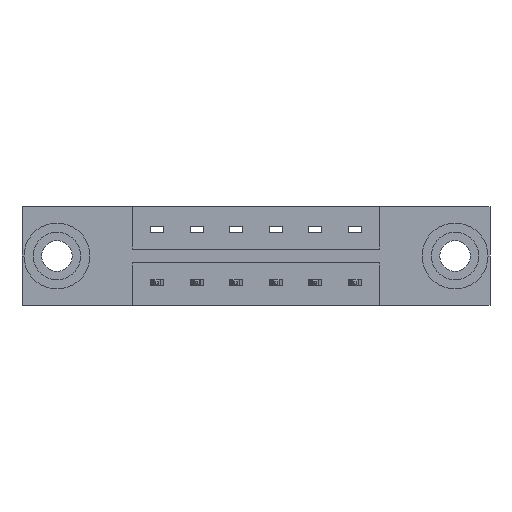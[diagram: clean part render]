
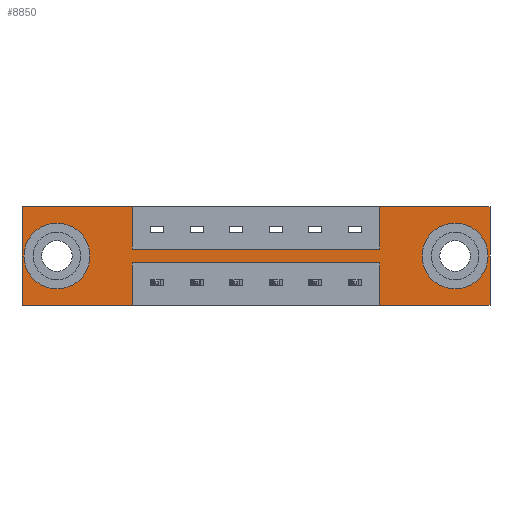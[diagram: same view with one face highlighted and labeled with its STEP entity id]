
A CAD part, front view. The second image highlights one B-rep face of the part: STEP entity #8850.
In plain terms, the highlighted planar face has unit normal (0, -1, 0).
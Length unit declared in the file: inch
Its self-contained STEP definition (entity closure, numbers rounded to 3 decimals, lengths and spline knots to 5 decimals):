
#190 = CARTESIAN_POINT ( 'NONE',  ( 0., 0., -0.375 ) ) ;
#404 = VECTOR ( 'NONE', #4801, 39.37008 ) ;
#410 = CARTESIAN_POINT ( 'NONE',  ( 1.3575, 0., -0.375 ) ) ;
#414 = CARTESIAN_POINT ( 'NONE',  ( 0.1325, 0., -0.2655 ) ) ;
#496 = EDGE_CURVE ( 'NONE', #5405, #872, #3525, .T. ) ;
#663 = CARTESIAN_POINT ( 'NONE',  ( 1.3575, 0., -0.214 ) ) ;
#673 = CIRCLE ( 'NONE', #7568, 0.078 ) ;
#729 = VERTEX_POINT ( 'NONE', #8102 ) ;
#759 = VERTEX_POINT ( 'NONE', #3220 ) ;
#762 = CARTESIAN_POINT ( 'NONE',  ( 1.3575, 0., 0. ) ) ;
#791 = LINE ( 'NONE', #9016, #7398 ) ;
#846 = DIRECTION ( 'NONE',  ( 1., 0., 0. ) ) ;
#872 = VERTEX_POINT ( 'NONE', #1295 ) ;
#899 = CARTESIAN_POINT ( 'NONE',  ( 0.4175, 0., -0.161 ) ) ;
#926 = EDGE_CURVE ( 'NONE', #759, #5905, #7261, .T. ) ;
#937 = EDGE_CURVE ( 'NONE', #6384, #6555, #5941, .T. ) ;
#1058 = AXIS2_PLACEMENT_3D ( 'NONE', #3857, #1076, #7950 ) ;
#1076 = DIRECTION ( 'NONE',  ( 0., 1., 0. ) ) ;
#1180 = CARTESIAN_POINT ( 'NONE',  ( 0., 0., -0.375 ) ) ;
#1185 = ORIENTED_EDGE ( 'NONE', *, *, #2031, .T. ) ;
#1244 = CARTESIAN_POINT ( 'NONE',  ( 0.1325, 0., -0.1875 ) ) ;
#1295 = CARTESIAN_POINT ( 'NONE',  ( 1.775, 0., -0.375 ) ) ;
#1306 = CARTESIAN_POINT ( 'NONE',  ( 0., 0., 0. ) ) ;
#1395 = VERTEX_POINT ( 'NONE', #899 ) ;
#1430 = CARTESIAN_POINT ( 'NONE',  ( 1.3575, 0., -0.161 ) ) ;
#1460 = ORIENTED_EDGE ( 'NONE', *, *, #926, .T. ) ;
#1486 = ORIENTED_EDGE ( 'NONE', *, *, #3105, .F. ) ;
#1494 = VECTOR ( 'NONE', #7271, 39.37008 ) ;
#1638 = CIRCLE ( 'NONE', #1058, 0.078 ) ;
#1701 = EDGE_CURVE ( 'NONE', #3191, #1395, #791, .T. ) ;
#1712 = DIRECTION ( 'NONE',  ( 0., 1., 0. ) ) ;
#1730 = EDGE_CURVE ( 'NONE', #2516, #3898, #7954, .T. ) ;
#1774 = EDGE_CURVE ( 'NONE', #4267, #6870, #8929, .T. ) ;
#1779 = CARTESIAN_POINT ( 'NONE',  ( 0.1325, 0., -0.1875 ) ) ;
#2002 = LINE ( 'NONE', #1180, #3651 ) ;
#2005 = DIRECTION ( 'NONE',  ( 0., 0., -1. ) ) ;
#2022 = CARTESIAN_POINT ( 'NONE',  ( 1.6425, 0., -0.2655 ) ) ;
#2031 = EDGE_CURVE ( 'NONE', #7749, #5658, #673, .T. ) ;
#2059 = ORIENTED_EDGE ( 'NONE', *, *, #5845, .T. ) ;
#2168 = ORIENTED_EDGE ( 'NONE', *, *, #1774, .F. ) ;
#2413 = CARTESIAN_POINT ( 'NONE',  ( 0.4175, 0., -0.214 ) ) ;
#2516 = VERTEX_POINT ( 'NONE', #5736 ) ;
#2550 = ORIENTED_EDGE ( 'NONE', *, *, #5203, .F. ) ;
#2601 = ORIENTED_EDGE ( 'NONE', *, *, #3678, .F. ) ;
#2663 = DIRECTION ( 'NONE',  ( 0., 1., 0. ) ) ;
#2703 = DIRECTION ( 'NONE',  ( 0., 0., 1. ) ) ;
#2781 = ORIENTED_EDGE ( 'NONE', *, *, #4868, .F. ) ;
#2834 = CARTESIAN_POINT ( 'NONE',  ( 0., 0., -0.375 ) ) ;
#2890 = AXIS2_PLACEMENT_3D ( 'NONE', #190, #8417, #2915 ) ;
#2915 = DIRECTION ( 'NONE',  ( 0., 0., -1. ) ) ;
#3105 = EDGE_CURVE ( 'NONE', #3347, #729, #7172, .T. ) ;
#3178 = DIRECTION ( 'NONE',  ( -1., 0., 0. ) ) ;
#3191 = VERTEX_POINT ( 'NONE', #4894 ) ;
#3196 = CARTESIAN_POINT ( 'NONE',  ( 1.775, 0., 0. ) ) ;
#3220 = CARTESIAN_POINT ( 'NONE',  ( 0.1325, 0., -0.1095 ) ) ;
#3228 = FACE_BOUND ( 'NONE', #6031, .T. ) ;
#3347 = VERTEX_POINT ( 'NONE', #410 ) ;
#3398 = CARTESIAN_POINT ( 'NONE',  ( 0.4175, 0., -0.214 ) ) ;
#3427 = ORIENTED_EDGE ( 'NONE', *, *, #1701, .F. ) ;
#3500 = DIRECTION ( 'NONE',  ( 1., 0., 0. ) ) ;
#3525 = LINE ( 'NONE', #8267, #6457 ) ;
#3616 = VECTOR ( 'NONE', #3178, 39.37008 ) ;
#3651 = VECTOR ( 'NONE', #8869, 39.37008 ) ;
#3678 = EDGE_CURVE ( 'NONE', #3898, #5405, #4124, .T. ) ;
#3685 = CARTESIAN_POINT ( 'NONE',  ( 1.6425, 0., -0.1875 ) ) ;
#3799 = VECTOR ( 'NONE', #6216, 39.37008 ) ;
#3857 = CARTESIAN_POINT ( 'NONE',  ( 1.6425, 0., -0.1875 ) ) ;
#3889 = VECTOR ( 'NONE', #3500, 39.37008 ) ;
#3898 = VERTEX_POINT ( 'NONE', #762 ) ;
#3922 = ORIENTED_EDGE ( 'NONE', *, *, #496, .F. ) ;
#4124 = LINE ( 'NONE', #7997, #1494 ) ;
#4267 = VERTEX_POINT ( 'NONE', #2834 ) ;
#4348 = VECTOR ( 'NONE', #6861, 39.37008 ) ;
#4504 = VECTOR ( 'NONE', #846, 39.37008 ) ;
#4527 = CARTESIAN_POINT ( 'NONE',  ( 0.4175, 0., -0.214 ) ) ;
#4772 = CARTESIAN_POINT ( 'NONE',  ( 0., 0., -0.375 ) ) ;
#4793 = AXIS2_PLACEMENT_3D ( 'NONE', #1244, #2663, #6089 ) ;
#4801 = DIRECTION ( 'NONE',  ( 0., 0., -1. ) ) ;
#4833 = ORIENTED_EDGE ( 'NONE', *, *, #937, .F. ) ;
#4868 = EDGE_CURVE ( 'NONE', #872, #3347, #2002, .T. ) ;
#4894 = CARTESIAN_POINT ( 'NONE',  ( 0.4175, 0., 0. ) ) ;
#5033 = ORIENTED_EDGE ( 'NONE', *, *, #1730, .F. ) ;
#5203 = EDGE_CURVE ( 'NONE', #1395, #2516, #8189, .T. ) ;
#5405 = VERTEX_POINT ( 'NONE', #3196 ) ;
#5658 = VERTEX_POINT ( 'NONE', #7627 ) ;
#5672 = VECTOR ( 'NONE', #8973, 39.37008 ) ;
#5736 = CARTESIAN_POINT ( 'NONE',  ( 1.3575, 0., -0.161 ) ) ;
#5845 = EDGE_CURVE ( 'NONE', #5658, #7749, #1638, .T. ) ;
#5905 = VERTEX_POINT ( 'NONE', #414 ) ;
#5940 = EDGE_CURVE ( 'NONE', #729, #6384, #6638, .T. ) ;
#5941 = LINE ( 'NONE', #3398, #404 ) ;
#5942 = CIRCLE ( 'NONE', #8532, 0.078 ) ;
#6031 = EDGE_LOOP ( 'NONE', ( #2059, #1185 ) ) ;
#6089 = DIRECTION ( 'NONE',  ( 0., 0., 1. ) ) ;
#6209 = DIRECTION ( 'NONE',  ( 0., 0., -1. ) ) ;
#6215 = ORIENTED_EDGE ( 'NONE', *, *, #8670, .F. ) ;
#6216 = DIRECTION ( 'NONE',  ( 0., 0., 1. ) ) ;
#6238 = CARTESIAN_POINT ( 'NONE',  ( 0., 0., 0. ) ) ;
#6384 = VERTEX_POINT ( 'NONE', #4527 ) ;
#6457 = VECTOR ( 'NONE', #6209, 39.37008 ) ;
#6555 = VERTEX_POINT ( 'NONE', #6888 ) ;
#6638 = LINE ( 'NONE', #2413, #3616 ) ;
#6640 = ORIENTED_EDGE ( 'NONE', *, *, #7853, .F. ) ;
#6653 = DIRECTION ( 'NONE',  ( 0., 0., 1. ) ) ;
#6762 = EDGE_LOOP ( 'NONE', ( #1486, #2781, #3922, #2601, #5033, #2550, #3427, #6215, #2168, #6640, #4833, #7526 ) ) ;
#6836 = ORIENTED_EDGE ( 'NONE', *, *, #7919, .T. ) ;
#6861 = DIRECTION ( 'NONE',  ( -1., 0., 0. ) ) ;
#6870 = VERTEX_POINT ( 'NONE', #6913 ) ;
#6888 = CARTESIAN_POINT ( 'NONE',  ( 0.4175, 0., -0.375 ) ) ;
#6913 = CARTESIAN_POINT ( 'NONE',  ( 0., 0., 0. ) ) ;
#6996 = PLANE ( 'NONE',  #2890 ) ;
#7172 = LINE ( 'NONE', #663, #3799 ) ;
#7212 = DIRECTION ( 'NONE',  ( 0., 1., 0. ) ) ;
#7261 = CIRCLE ( 'NONE', #4793, 0.078 ) ;
#7271 = DIRECTION ( 'NONE',  ( 1., 0., 0. ) ) ;
#7352 = FACE_OUTER_BOUND ( 'NONE', #6762, .T. ) ;
#7398 = VECTOR ( 'NONE', #2005, 39.37008 ) ;
#7481 = LINE ( 'NONE', #4772, #4348 ) ;
#7526 = ORIENTED_EDGE ( 'NONE', *, *, #5940, .F. ) ;
#7568 = AXIS2_PLACEMENT_3D ( 'NONE', #3685, #7212, #7907 ) ;
#7627 = CARTESIAN_POINT ( 'NONE',  ( 1.6425, 0., -0.1095 ) ) ;
#7724 = EDGE_LOOP ( 'NONE', ( #1460, #6836 ) ) ;
#7749 = VERTEX_POINT ( 'NONE', #2022 ) ;
#7807 = FACE_BOUND ( 'NONE', #7724, .T. ) ;
#7853 = EDGE_CURVE ( 'NONE', #6555, #4267, #7481, .T. ) ;
#7907 = DIRECTION ( 'NONE',  ( 0., 0., -1. ) ) ;
#7919 = EDGE_CURVE ( 'NONE', #5905, #759, #5942, .T. ) ;
#7950 = DIRECTION ( 'NONE',  ( 0., 0., -1. ) ) ;
#7954 = LINE ( 'NONE', #1430, #8265 ) ;
#7997 = CARTESIAN_POINT ( 'NONE',  ( 0., 0., 0. ) ) ;
#8102 = CARTESIAN_POINT ( 'NONE',  ( 1.3575, 0., -0.214 ) ) ;
#8112 = LINE ( 'NONE', #1306, #3889 ) ;
#8189 = LINE ( 'NONE', #8451, #4504 ) ;
#8265 = VECTOR ( 'NONE', #2703, 39.37008 ) ;
#8267 = CARTESIAN_POINT ( 'NONE',  ( 1.775, 0., 0. ) ) ;
#8417 = DIRECTION ( 'NONE',  ( 0., -1., 0. ) ) ;
#8451 = CARTESIAN_POINT ( 'NONE',  ( 0.4175, 0., -0.161 ) ) ;
#8532 = AXIS2_PLACEMENT_3D ( 'NONE', #1779, #1712, #6653 ) ;
#8670 = EDGE_CURVE ( 'NONE', #6870, #3191, #8112, .T. ) ;
#8850 = ADVANCED_FACE ( 'NONE', ( #3228, #7807, #7352 ), #6996, .T. ) ;
#8869 = DIRECTION ( 'NONE',  ( -1., 0., 0. ) ) ;
#8929 = LINE ( 'NONE', #6238, #5672 ) ;
#8973 = DIRECTION ( 'NONE',  ( 0., 0., 1. ) ) ;
#9016 = CARTESIAN_POINT ( 'NONE',  ( 0.4175, 0., -0.161 ) ) ;
